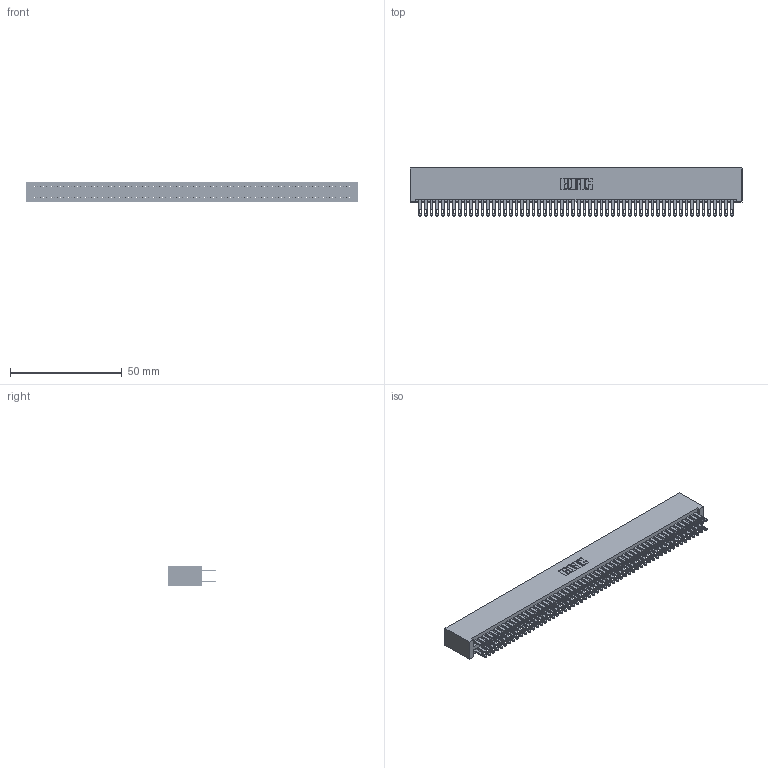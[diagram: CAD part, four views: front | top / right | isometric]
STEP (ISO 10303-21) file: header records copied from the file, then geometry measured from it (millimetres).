
FILE_DESCRIPTION (( 'STEP AP203' ), '1' );
FILE_NAME ('345-112-500-201.STEP', '2018-10-07T13:05:34', ( '' ), ( '' ), 'SwSTEP 2.0', 'SolidWorks 2016', '' );
FILE_SCHEMA (( 'CONFIG_CONTROL_DESIGN' ));
Length unit declared in the file: inch
Products named in the file (3): 345-112-500-201; 345-292-001_345-293-100; 345 Part_No Mounting Lugs
Assembly tree (113 placements, depth 2):
  345-112-500-201
    345 Part_No Mounting Lugs
    345-292-001_345-293-100  x112
Bounding box: 148.84 x 21.51 x 9.4 mm (x, y, z)
Volume: 15547 mm3; surface area: 24697.8 mm2
Topology: 113 solids, 113 shells, 5270 faces, 16109 edges, 10738 vertices
Faces by surface type: plane 3100, cylinder 2170
Entity records: 41707 total; most frequent: CARTESIAN_POINT 6976, ORIENTED_EDGE 6910, DIRECTION 6131, EDGE_CURVE 3455, LINE 3103, VECTOR 3103, VERTEX_POINT 2302, AXIS2_PLACEMENT_3D 1514
